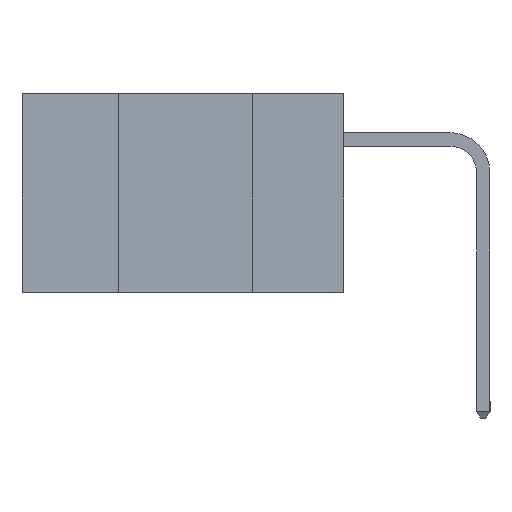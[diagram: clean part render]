
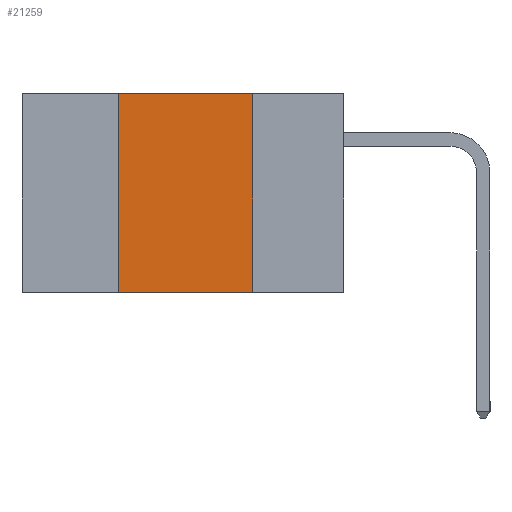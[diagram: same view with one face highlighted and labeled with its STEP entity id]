
A CAD part, left-side view. The second image highlights one B-rep face of the part: STEP entity #21259.
In plain terms, the highlighted planar face has unit normal (-1, 0, 0).
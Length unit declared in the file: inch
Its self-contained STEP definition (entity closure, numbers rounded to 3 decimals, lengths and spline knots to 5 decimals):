
#139 = CARTESIAN_POINT ( 'NONE',  ( 0., 0.17, -0.37 ) ) ;
#683 = EDGE_LOOP ( 'NONE', ( #1414, #5604, #25244, #7629 ) ) ;
#857 = DIRECTION ( 'NONE',  ( 0., -1., 0. ) ) ;
#999 = EDGE_CURVE ( 'NONE', #24473, #13824, #20040, .T. ) ;
#1218 = CARTESIAN_POINT ( 'NONE',  ( 0., 0.6, -0.37 ) ) ;
#1414 = ORIENTED_EDGE ( 'NONE', *, *, #7921, .F. ) ;
#1999 = CARTESIAN_POINT ( 'NONE',  ( 0., 0.42, -0.37 ) ) ;
#3061 = DIRECTION ( 'NONE',  ( 0., -1., 0. ) ) ;
#3916 = CARTESIAN_POINT ( 'NONE',  ( 0., 0.17, 0. ) ) ;
#4222 = CARTESIAN_POINT ( 'NONE',  ( 0., 0.6, 0. ) ) ;
#4711 = VERTEX_POINT ( 'NONE', #24620 ) ;
#4999 = VERTEX_POINT ( 'NONE', #3916 ) ;
#5312 = DIRECTION ( 'NONE',  ( 0., 0., -1. ) ) ;
#5604 = ORIENTED_EDGE ( 'NONE', *, *, #11634, .F. ) ;
#5929 = LINE ( 'NONE', #10259, #21623 ) ;
#6048 = FACE_OUTER_BOUND ( 'NONE', #683, .T. ) ;
#6165 = DIRECTION ( 'NONE',  ( 1., 0., 0. ) ) ;
#6292 = EDGE_CURVE ( 'NONE', #24473, #4711, #5929, .T. ) ;
#7629 = ORIENTED_EDGE ( 'NONE', *, *, #999, .T. ) ;
#7921 = EDGE_CURVE ( 'NONE', #4999, #13824, #16023, .T. ) ;
#8695 = CARTESIAN_POINT ( 'NONE',  ( 0., 0.6, 0. ) ) ;
#10171 = VECTOR ( 'NONE', #5312, 39.37008 ) ;
#10259 = CARTESIAN_POINT ( 'NONE',  ( 0., 0.42, -0.37 ) ) ;
#11634 = EDGE_CURVE ( 'NONE', #4711, #4999, #13660, .T. ) ;
#13660 = LINE ( 'NONE', #8695, #18316 ) ;
#13824 = VERTEX_POINT ( 'NONE', #139 ) ;
#14790 = VECTOR ( 'NONE', #3061, 39.37008 ) ;
#14984 = CARTESIAN_POINT ( 'NONE',  ( 0., 0.17, -0.37 ) ) ;
#15987 = PLANE ( 'NONE',  #16680 ) ;
#16023 = LINE ( 'NONE', #14984, #10171 ) ;
#16680 = AXIS2_PLACEMENT_3D ( 'NONE', #4222, #6165, #19931 ) ;
#18316 = VECTOR ( 'NONE', #857, 39.37008 ) ;
#19931 = DIRECTION ( 'NONE',  ( 0., 0., -1. ) ) ;
#20040 = LINE ( 'NONE', #1218, #14790 ) ;
#21259 = ADVANCED_FACE ( 'NONE', ( #6048 ), #15987, .F. ) ;
#21623 = VECTOR ( 'NONE', #22050, 39.37008 ) ;
#22050 = DIRECTION ( 'NONE',  ( 0., 0., 1. ) ) ;
#24473 = VERTEX_POINT ( 'NONE', #1999 ) ;
#24620 = CARTESIAN_POINT ( 'NONE',  ( 0., 0.42, 0. ) ) ;
#25244 = ORIENTED_EDGE ( 'NONE', *, *, #6292, .F. ) ;
